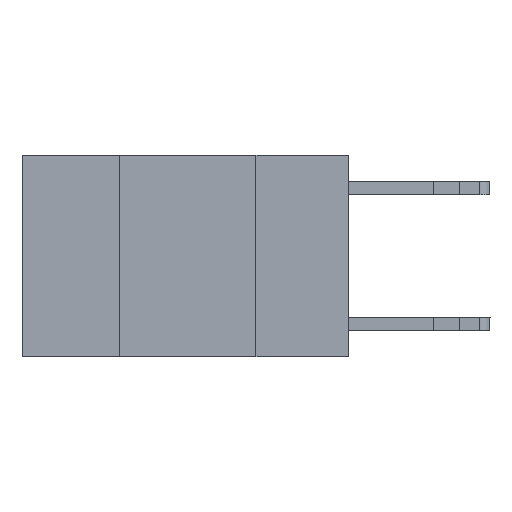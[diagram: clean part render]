
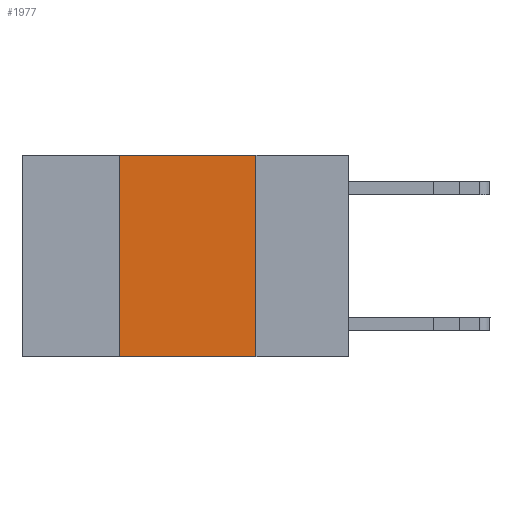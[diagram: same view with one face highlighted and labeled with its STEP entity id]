
A CAD part, left-side view. The second image highlights one B-rep face of the part: STEP entity #1977.
In plain terms, the highlighted planar face has unit normal (-1, 0, 0).
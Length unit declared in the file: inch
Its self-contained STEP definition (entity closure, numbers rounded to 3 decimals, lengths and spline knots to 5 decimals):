
#455 = CARTESIAN_POINT ( 'NONE',  ( 0., 0.17, -0.37 ) ) ;
#1244 = EDGE_CURVE ( 'NONE', #6896, #3626, #10966, .T. ) ;
#1474 = CARTESIAN_POINT ( 'NONE',  ( 0., 0.42, 0. ) ) ;
#1674 = PLANE ( 'NONE',  #2410 ) ;
#1954 = CARTESIAN_POINT ( 'NONE',  ( 0., 0.42, 0. ) ) ;
#1977 = ADVANCED_FACE ( 'NONE', ( #5470 ), #1674, .F. ) ;
#2410 = AXIS2_PLACEMENT_3D ( 'NONE', #4963, #4487, #3563 ) ;
#2538 = VECTOR ( 'NONE', #10581, 39.37008 ) ;
#2643 = LINE ( 'NONE', #6013, #9598 ) ;
#3216 = EDGE_CURVE ( 'NONE', #3626, #4958, #4978, .T. ) ;
#3563 = DIRECTION ( 'NONE',  ( 0., 0., -1. ) ) ;
#3626 = VERTEX_POINT ( 'NONE', #8750 ) ;
#4049 = ORIENTED_EDGE ( 'NONE', *, *, #7313, .F. ) ;
#4487 = DIRECTION ( 'NONE',  ( 1., 0., 0. ) ) ;
#4958 = VERTEX_POINT ( 'NONE', #455 ) ;
#4963 = CARTESIAN_POINT ( 'NONE',  ( 0., 0.6, 0. ) ) ;
#4978 = LINE ( 'NONE', #10115, #2538 ) ;
#5470 = FACE_OUTER_BOUND ( 'NONE', #10652, .T. ) ;
#5933 = ORIENTED_EDGE ( 'NONE', *, *, #11017, .T. ) ;
#6013 = CARTESIAN_POINT ( 'NONE',  ( 0., 0.6, -0.37 ) ) ;
#6102 = VERTEX_POINT ( 'NONE', #6872 ) ;
#6330 = VECTOR ( 'NONE', #9133, 39.37008 ) ;
#6872 = CARTESIAN_POINT ( 'NONE',  ( 0., 0.42, -0.37 ) ) ;
#6896 = VERTEX_POINT ( 'NONE', #1474 ) ;
#6932 = ORIENTED_EDGE ( 'NONE', *, *, #3216, .F. ) ;
#7313 = EDGE_CURVE ( 'NONE', #6102, #6896, #9184, .T. ) ;
#7996 = CARTESIAN_POINT ( 'NONE',  ( 0., 0.6, 0. ) ) ;
#8330 = DIRECTION ( 'NONE',  ( 0., 0., 1. ) ) ;
#8750 = CARTESIAN_POINT ( 'NONE',  ( 0., 0.17, 0. ) ) ;
#9133 = DIRECTION ( 'NONE',  ( 0., -1., 0. ) ) ;
#9184 = LINE ( 'NONE', #1954, #9714 ) ;
#9598 = VECTOR ( 'NONE', #11212, 39.37008 ) ;
#9702 = ORIENTED_EDGE ( 'NONE', *, *, #1244, .F. ) ;
#9714 = VECTOR ( 'NONE', #8330, 39.37008 ) ;
#10115 = CARTESIAN_POINT ( 'NONE',  ( 0., 0.17, 0. ) ) ;
#10581 = DIRECTION ( 'NONE',  ( 0., 0., -1. ) ) ;
#10652 = EDGE_LOOP ( 'NONE', ( #6932, #9702, #4049, #5933 ) ) ;
#10966 = LINE ( 'NONE', #7996, #6330 ) ;
#11017 = EDGE_CURVE ( 'NONE', #6102, #4958, #2643, .T. ) ;
#11212 = DIRECTION ( 'NONE',  ( 0., -1., 0. ) ) ;
